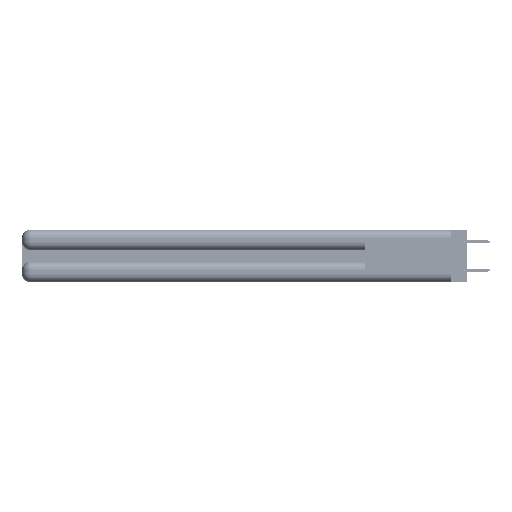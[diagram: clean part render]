
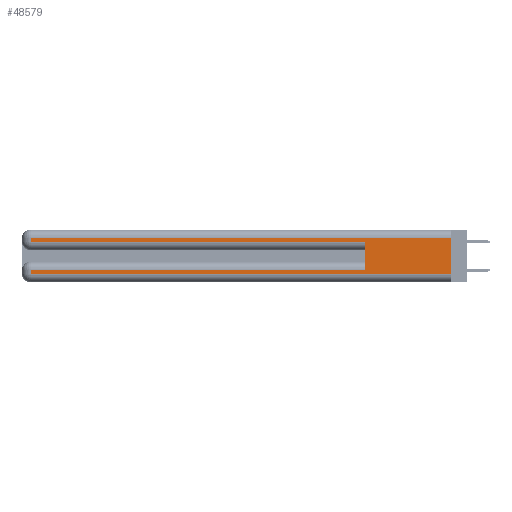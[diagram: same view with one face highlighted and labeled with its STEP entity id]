
A CAD part, left-side view. The second image highlights one B-rep face of the part: STEP entity #48579.
In plain terms, the highlighted planar face has unit normal (-1, 0, 0).
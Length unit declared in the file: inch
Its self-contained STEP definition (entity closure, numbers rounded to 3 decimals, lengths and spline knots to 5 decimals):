
#301 = LINE ( 'NONE', #10634, #11947 ) ;
#424 = EDGE_CURVE ( 'NONE', #53534, #12192, #9197, .T. ) ;
#484 = CARTESIAN_POINT ( 'NONE',  ( 0., 0., 0.285 ) ) ;
#1953 = EDGE_CURVE ( 'NONE', #50011, #9388, #42236, .T. ) ;
#6095 = VERTEX_POINT ( 'NONE', #37359 ) ;
#6819 = DIRECTION ( 'NONE',  ( 0., 0., 1. ) ) ;
#8057 = CARTESIAN_POINT ( 'NONE',  ( 0., 0., 0.31 ) ) ;
#9117 = VERTEX_POINT ( 'NONE', #15302 ) ;
#9197 = LINE ( 'NONE', #484, #44089 ) ;
#9388 = VERTEX_POINT ( 'NONE', #43014 ) ;
#9782 = LINE ( 'NONE', #50136, #31658 ) ;
#10634 = CARTESIAN_POINT ( 'NONE',  ( 0., 0., 0.06 ) ) ;
#11947 = VECTOR ( 'NONE', #32411, 39.37008 ) ;
#12192 = VERTEX_POINT ( 'NONE', #15436 ) ;
#12912 = EDGE_CURVE ( 'NONE', #39424, #9117, #16180, .T. ) ;
#13118 = EDGE_LOOP ( 'NONE', ( #30877, #54920, #22862, #17048, #46001, #55316, #30455, #27123 ) ) ;
#14720 = CARTESIAN_POINT ( 'NONE',  ( 0., 0., 0.31 ) ) ;
#15302 = CARTESIAN_POINT ( 'NONE',  ( 0., 2.94, 0.06 ) ) ;
#15436 = CARTESIAN_POINT ( 'NONE',  ( 0., 0.6, 0.285 ) ) ;
#16180 = LINE ( 'NONE', #28756, #26452 ) ;
#16634 = CARTESIAN_POINT ( 'NONE',  ( 0., 0., 0.37 ) ) ;
#16962 = CARTESIAN_POINT ( 'NONE',  ( 0., 0., 0.37 ) ) ;
#17048 = ORIENTED_EDGE ( 'NONE', *, *, #424, .T. ) ;
#19327 = EDGE_CURVE ( 'NONE', #28227, #39424, #9782, .T. ) ;
#20982 = VECTOR ( 'NONE', #51069, 39.37008 ) ;
#21015 = DIRECTION ( 'NONE',  ( 0., 0., -1. ) ) ;
#21322 = DIRECTION ( 'NONE',  ( 0., 0., -1. ) ) ;
#21821 = VECTOR ( 'NONE', #6819, 39.37008 ) ;
#22360 = LINE ( 'NONE', #46667, #20982 ) ;
#22457 = AXIS2_PLACEMENT_3D ( 'NONE', #16962, #47530, #21322 ) ;
#22862 = ORIENTED_EDGE ( 'NONE', *, *, #51507, .T. ) ;
#24184 = DIRECTION ( 'NONE',  ( 0., 0., -1. ) ) ;
#26452 = VECTOR ( 'NONE', #24184, 39.37008 ) ;
#27123 = ORIENTED_EDGE ( 'NONE', *, *, #47085, .T. ) ;
#28227 = VERTEX_POINT ( 'NONE', #38212 ) ;
#28346 = DIRECTION ( 'NONE',  ( 0., 1., 0. ) ) ;
#28756 = CARTESIAN_POINT ( 'NONE',  ( 0., 2.94, 0.37 ) ) ;
#30455 = ORIENTED_EDGE ( 'NONE', *, *, #12912, .T. ) ;
#30877 = ORIENTED_EDGE ( 'NONE', *, *, #42483, .F. ) ;
#31085 = DIRECTION ( 'NONE',  ( 0., -1., 0. ) ) ;
#31554 = VECTOR ( 'NONE', #21015, 39.37008 ) ;
#31658 = VECTOR ( 'NONE', #28346, 39.37008 ) ;
#32411 = DIRECTION ( 'NONE',  ( 0., -1., 0. ) ) ;
#32919 = LINE ( 'NONE', #16634, #31554 ) ;
#35339 = EDGE_CURVE ( 'NONE', #28227, #12192, #55303, .T. ) ;
#37359 = CARTESIAN_POINT ( 'NONE',  ( 0., 0., 0.06 ) ) ;
#37409 = CARTESIAN_POINT ( 'NONE',  ( 0., 0.6, 0.145 ) ) ;
#38212 = CARTESIAN_POINT ( 'NONE',  ( 0., 0.6, 0.085 ) ) ;
#39424 = VERTEX_POINT ( 'NONE', #43689 ) ;
#40884 = VECTOR ( 'NONE', #51820, 39.37008 ) ;
#42236 = LINE ( 'NONE', #8057, #40884 ) ;
#42483 = EDGE_CURVE ( 'NONE', #50011, #6095, #32919, .T. ) ;
#42513 = CARTESIAN_POINT ( 'NONE',  ( 0., 2.94, 0.285 ) ) ;
#42547 = FACE_OUTER_BOUND ( 'NONE', #13118, .T. ) ;
#43014 = CARTESIAN_POINT ( 'NONE',  ( 0., 2.94, 0.31 ) ) ;
#43154 = PLANE ( 'NONE',  #22457 ) ;
#43689 = CARTESIAN_POINT ( 'NONE',  ( 0., 2.94, 0.085 ) ) ;
#44089 = VECTOR ( 'NONE', #31085, 39.37008 ) ;
#46001 = ORIENTED_EDGE ( 'NONE', *, *, #35339, .F. ) ;
#46667 = CARTESIAN_POINT ( 'NONE',  ( 0., 2.94, 0.37 ) ) ;
#47085 = EDGE_CURVE ( 'NONE', #9117, #6095, #301, .T. ) ;
#47530 = DIRECTION ( 'NONE',  ( 1., 0., 0. ) ) ;
#48579 = ADVANCED_FACE ( 'NONE', ( #42547 ), #43154, .F. ) ;
#50011 = VERTEX_POINT ( 'NONE', #14720 ) ;
#50136 = CARTESIAN_POINT ( 'NONE',  ( 0., 0., 0.085 ) ) ;
#51069 = DIRECTION ( 'NONE',  ( 0., 0., -1. ) ) ;
#51507 = EDGE_CURVE ( 'NONE', #9388, #53534, #22360, .T. ) ;
#51820 = DIRECTION ( 'NONE',  ( 0., 1., 0. ) ) ;
#53534 = VERTEX_POINT ( 'NONE', #42513 ) ;
#54920 = ORIENTED_EDGE ( 'NONE', *, *, #1953, .T. ) ;
#55303 = LINE ( 'NONE', #37409, #21821 ) ;
#55316 = ORIENTED_EDGE ( 'NONE', *, *, #19327, .T. ) ;
